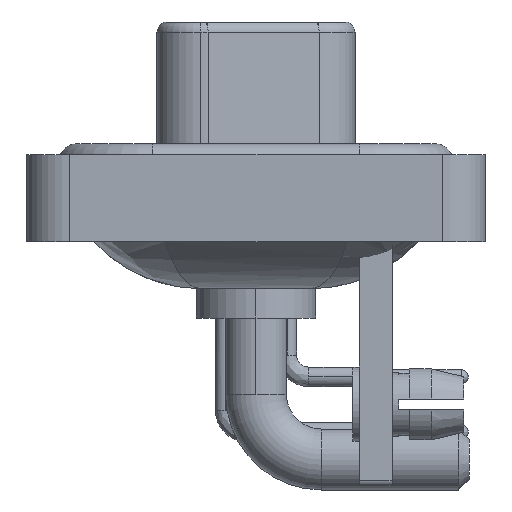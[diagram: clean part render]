
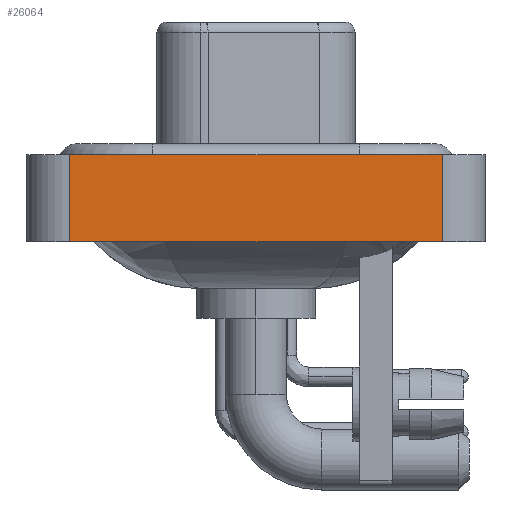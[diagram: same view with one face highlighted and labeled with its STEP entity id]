
A CAD part, left-side view. The second image highlights one B-rep face of the part: STEP entity #26064.
In plain terms, the highlighted planar face has unit normal (-1, 0, 0).
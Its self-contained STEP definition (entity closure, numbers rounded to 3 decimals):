
#1963 = LINE ( 'NONE', #25319, #13002 ) ;
#2766 = CARTESIAN_POINT ( 'NONE',  ( -7.35, 8.55, 0.4 ) ) ;
#4130 = VERTEX_POINT ( 'NONE', #15960 ) ;
#4266 = CARTESIAN_POINT ( 'NONE',  ( -7.35, -8.55, -3.6 ) ) ;
#4395 = LINE ( 'NONE', #14070, #22137 ) ;
#5748 = ORIENTED_EDGE ( 'NONE', *, *, #17508, .T. ) ;
#6698 = CARTESIAN_POINT ( 'NONE',  ( -7.35, -8.55, 0.4 ) ) ;
#7370 = CARTESIAN_POINT ( 'NONE',  ( -7.35, 8.55, -3.6 ) ) ;
#8211 = VECTOR ( 'NONE', #11949, 1000. ) ;
#8964 = EDGE_CURVE ( 'NONE', #4130, #29913, #23892, .T. ) ;
#9276 = DIRECTION ( 'NONE',  ( 0., -1., 0. ) ) ;
#9779 = VECTOR ( 'NONE', #16905, 1000. ) ;
#10409 = VERTEX_POINT ( 'NONE', #6698 ) ;
#10569 = FACE_OUTER_BOUND ( 'NONE', #26472, .T. ) ;
#10728 = DIRECTION ( 'NONE',  ( -1., 0., 0. ) ) ;
#11047 = ORIENTED_EDGE ( 'NONE', *, *, #25217, .F. ) ;
#11474 = LINE ( 'NONE', #4266, #8211 ) ;
#11517 = ORIENTED_EDGE ( 'NONE', *, *, #15818, .T. ) ;
#11949 = DIRECTION ( 'NONE',  ( 0., -1., 0. ) ) ;
#13002 = VECTOR ( 'NONE', #9276, 1000. ) ;
#14070 = CARTESIAN_POINT ( 'NONE',  ( -7.35, -8.55, -3.6 ) ) ;
#15818 = EDGE_CURVE ( 'NONE', #4130, #21217, #11474, .T. ) ;
#15960 = CARTESIAN_POINT ( 'NONE',  ( -7.35, 8.55, -3.6 ) ) ;
#16905 = DIRECTION ( 'NONE',  ( 0., 0., 1. ) ) ;
#17508 = EDGE_CURVE ( 'NONE', #21217, #10409, #4395, .T. ) ;
#18319 = AXIS2_PLACEMENT_3D ( 'NONE', #24897, #10728, #22710 ) ;
#19282 = CARTESIAN_POINT ( 'NONE',  ( -7.35, -8.55, -3.6 ) ) ;
#20057 = PLANE ( 'NONE',  #18319 ) ;
#21217 = VERTEX_POINT ( 'NONE', #19282 ) ;
#22137 = VECTOR ( 'NONE', #30271, 1000. ) ;
#22710 = DIRECTION ( 'NONE',  ( 0., 0., 1. ) ) ;
#23892 = LINE ( 'NONE', #7370, #9779 ) ;
#23999 = ORIENTED_EDGE ( 'NONE', *, *, #8964, .F. ) ;
#24897 = CARTESIAN_POINT ( 'NONE',  ( -7.35, -8.55, -3.6 ) ) ;
#25217 = EDGE_CURVE ( 'NONE', #29913, #10409, #1963, .T. ) ;
#25319 = CARTESIAN_POINT ( 'NONE',  ( -7.35, -8.55, 0.4 ) ) ;
#26064 = ADVANCED_FACE ( 'NONE', ( #10569 ), #20057, .T. ) ;
#26472 = EDGE_LOOP ( 'NONE', ( #5748, #11047, #23999, #11517 ) ) ;
#29913 = VERTEX_POINT ( 'NONE', #2766 ) ;
#30271 = DIRECTION ( 'NONE',  ( 0., 0., 1. ) ) ;
